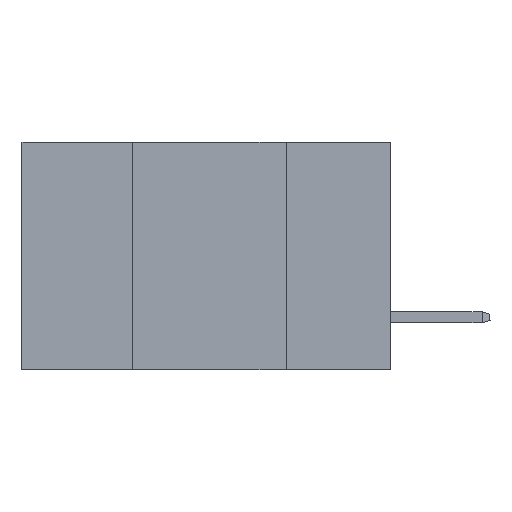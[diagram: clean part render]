
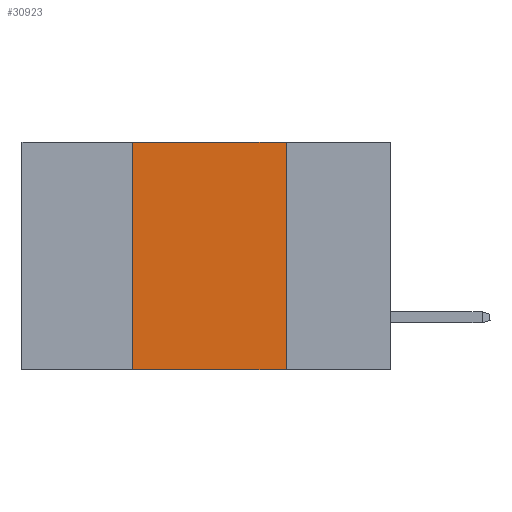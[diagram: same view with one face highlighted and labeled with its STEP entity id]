
A CAD part, left-side view. The second image highlights one B-rep face of the part: STEP entity #30923.
In plain terms, the highlighted planar face has unit normal (-1, 0, 0).
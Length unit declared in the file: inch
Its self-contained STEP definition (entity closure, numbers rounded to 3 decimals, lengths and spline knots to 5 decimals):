
#1575 = LINE ( 'NONE', #10406, #34130 ) ;
#2490 = ORIENTED_EDGE ( 'NONE', *, *, #35690, .F. ) ;
#2492 = VECTOR ( 'NONE', #30013, 39.37008 ) ;
#5342 = LINE ( 'NONE', #24403, #37402 ) ;
#6136 = AXIS2_PLACEMENT_3D ( 'NONE', #36828, #40354, #27147 ) ;
#7165 = VERTEX_POINT ( 'NONE', #13014 ) ;
#7860 = EDGE_CURVE ( 'NONE', #34354, #7165, #39819, .T. ) ;
#10406 = CARTESIAN_POINT ( 'NONE',  ( 0., 0.42, 0. ) ) ;
#10435 = VERTEX_POINT ( 'NONE', #20045 ) ;
#11621 = ORIENTED_EDGE ( 'NONE', *, *, #38280, .T. ) ;
#13014 = CARTESIAN_POINT ( 'NONE',  ( 0., 0.17, -0.37 ) ) ;
#13497 = PLANE ( 'NONE',  #6136 ) ;
#15177 = EDGE_LOOP ( 'NONE', ( #17437, #39432, #2490, #11621 ) ) ;
#16172 = CARTESIAN_POINT ( 'NONE',  ( 0., 0.42, 0. ) ) ;
#16628 = CARTESIAN_POINT ( 'NONE',  ( 0., 0.17, 0. ) ) ;
#17437 = ORIENTED_EDGE ( 'NONE', *, *, #7860, .F. ) ;
#20045 = CARTESIAN_POINT ( 'NONE',  ( 0., 0.42, -0.37 ) ) ;
#20615 = DIRECTION ( 'NONE',  ( 0., -1., 0. ) ) ;
#24403 = CARTESIAN_POINT ( 'NONE',  ( 0., 0.6, 0. ) ) ;
#26493 = VERTEX_POINT ( 'NONE', #16172 ) ;
#27147 = DIRECTION ( 'NONE',  ( 0., 0., -1. ) ) ;
#27582 = VECTOR ( 'NONE', #30667, 39.37008 ) ;
#30013 = DIRECTION ( 'NONE',  ( 0., 0., -1. ) ) ;
#30629 = FACE_OUTER_BOUND ( 'NONE', #15177, .T. ) ;
#30667 = DIRECTION ( 'NONE',  ( 0., -1., 0. ) ) ;
#30923 = ADVANCED_FACE ( 'NONE', ( #30629 ), #13497, .F. ) ;
#34032 = DIRECTION ( 'NONE',  ( 0., 0., 1. ) ) ;
#34130 = VECTOR ( 'NONE', #34032, 39.37008 ) ;
#34354 = VERTEX_POINT ( 'NONE', #36591 ) ;
#35690 = EDGE_CURVE ( 'NONE', #10435, #26493, #1575, .T. ) ;
#36591 = CARTESIAN_POINT ( 'NONE',  ( 0., 0.17, 0. ) ) ;
#36828 = CARTESIAN_POINT ( 'NONE',  ( 0., 0.6, 0. ) ) ;
#37402 = VECTOR ( 'NONE', #20615, 39.37008 ) ;
#38280 = EDGE_CURVE ( 'NONE', #10435, #7165, #43281, .T. ) ;
#39432 = ORIENTED_EDGE ( 'NONE', *, *, #43010, .F. ) ;
#39819 = LINE ( 'NONE', #16628, #2492 ) ;
#40354 = DIRECTION ( 'NONE',  ( 1., 0., 0. ) ) ;
#41214 = CARTESIAN_POINT ( 'NONE',  ( 0., 0.6, -0.37 ) ) ;
#43010 = EDGE_CURVE ( 'NONE', #26493, #34354, #5342, .T. ) ;
#43281 = LINE ( 'NONE', #41214, #27582 ) ;
